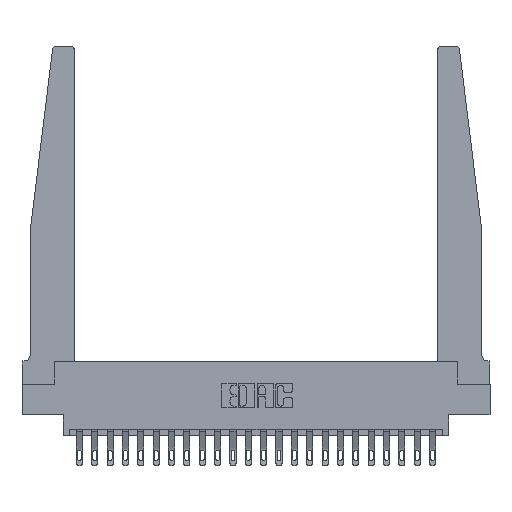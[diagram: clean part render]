
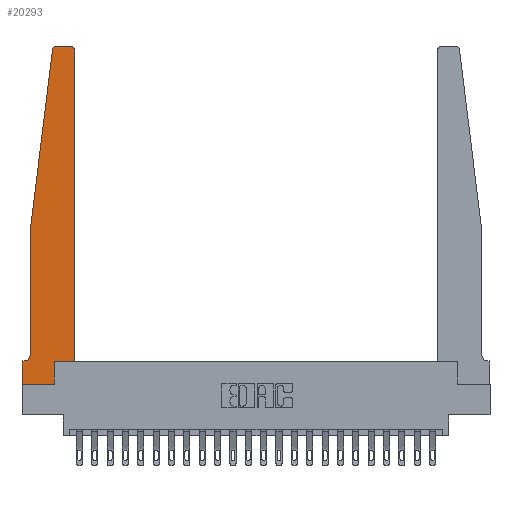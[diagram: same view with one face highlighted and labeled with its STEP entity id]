
A CAD part, top view. The second image highlights one B-rep face of the part: STEP entity #20293.
In plain terms, the highlighted planar face has unit normal (0, 0, 1).
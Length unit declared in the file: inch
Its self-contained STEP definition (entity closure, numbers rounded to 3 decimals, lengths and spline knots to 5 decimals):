
#299 = CIRCLE ( 'NONE', #3217, 0.03 ) ;
#361 = ORIENTED_EDGE ( 'NONE', *, *, #21332, .T. ) ;
#588 = VECTOR ( 'NONE', #3275, 39.37008 ) ;
#765 = LINE ( 'NONE', #5804, #19380 ) ;
#890 = EDGE_CURVE ( 'NONE', #10286, #17745, #2139, .T. ) ;
#1192 = VERTEX_POINT ( 'NONE', #19790 ) ;
#1317 = LINE ( 'NONE', #15060, #19360 ) ;
#1356 = AXIS2_PLACEMENT_3D ( 'NONE', #9595, #22176, #11411 ) ;
#1451 = DIRECTION ( 'NONE',  ( 0., 0., 1. ) ) ;
#1475 = CARTESIAN_POINT ( 'NONE',  ( 0.065, 1.25, 0.37 ) ) ;
#1739 = CARTESIAN_POINT ( 'NONE',  ( 0.425, 0.18, 0.37 ) ) ;
#1819 = ORIENTED_EDGE ( 'NONE', *, *, #6641, .T. ) ;
#1929 = CARTESIAN_POINT ( 'NONE',  ( 0.395, 2.75, 0.37 ) ) ;
#2139 = CIRCLE ( 'NONE', #16858, 0.05 ) ;
#3217 = AXIS2_PLACEMENT_3D ( 'NONE', #12265, #1451, #14056 ) ;
#3275 = DIRECTION ( 'NONE',  ( 0., -1., 0. ) ) ;
#3302 = CARTESIAN_POINT ( 'NONE',  ( 0.25, 2.75, 0.37 ) ) ;
#3959 = CARTESIAN_POINT ( 'NONE',  ( 0.065, 1.25, 0.37 ) ) ;
#4139 = CARTESIAN_POINT ( 'NONE',  ( 0.065, 0.2375, 0.37 ) ) ;
#4265 = DIRECTION ( 'NONE',  ( 0., 0., -1. ) ) ;
#4546 = EDGE_CURVE ( 'NONE', #10987, #20849, #12715, .T. ) ;
#4805 = ORIENTED_EDGE ( 'NONE', *, *, #10720, .T. ) ;
#4909 = VERTEX_POINT ( 'NONE', #11086 ) ;
#4997 = CARTESIAN_POINT ( 'NONE',  ( 0.27653, 2.75, 0.37 ) ) ;
#5639 = EDGE_LOOP ( 'NONE', ( #9806, #10664, #12303, #15102, #15524, #12689, #11533, #22842, #361, #4805, #1819, #17310 ) ) ;
#5682 = LINE ( 'NONE', #3302, #18344 ) ;
#5761 = LINE ( 'NONE', #9422, #9961 ) ;
#5804 = CARTESIAN_POINT ( 'NONE',  ( 0.2605, 0.18, 0.37 ) ) ;
#6040 = CARTESIAN_POINT ( 'NONE',  ( 0.2605, 0., 0.37 ) ) ;
#6432 = VECTOR ( 'NONE', #16168, 39.37008 ) ;
#6503 = CARTESIAN_POINT ( 'NONE',  ( 0., 0., 0.37 ) ) ;
#6641 = EDGE_CURVE ( 'NONE', #4909, #10987, #19247, .T. ) ;
#6982 = LINE ( 'NONE', #1739, #6432 ) ;
#7587 = DIRECTION ( 'NONE',  ( 0., 1., 0. ) ) ;
#7610 = EDGE_CURVE ( 'NONE', #13910, #10286, #20336, .T. ) ;
#7675 = DIRECTION ( 'NONE',  ( -1., 0., 0. ) ) ;
#7813 = DIRECTION ( 'NONE',  ( 0., 1., 0. ) ) ;
#7872 = DIRECTION ( 'NONE',  ( 1., 0., 0. ) ) ;
#8083 = LINE ( 'NONE', #10936, #17113 ) ;
#8285 = VERTEX_POINT ( 'NONE', #10668 ) ;
#8315 = CARTESIAN_POINT ( 'NONE',  ( 0., 0.1875, 0.37 ) ) ;
#8373 = AXIS2_PLACEMENT_3D ( 'NONE', #20166, #21979, #11200 ) ;
#9387 = PLANE ( 'NONE',  #8373 ) ;
#9422 = CARTESIAN_POINT ( 'NONE',  ( 0.065, 0.1875, 0.37 ) ) ;
#9595 = CARTESIAN_POINT ( 'NONE',  ( 0.395, 2.72, 0.37 ) ) ;
#9806 = ORIENTED_EDGE ( 'NONE', *, *, #16970, .T. ) ;
#9961 = VECTOR ( 'NONE', #7675, 39.37008 ) ;
#10286 = VERTEX_POINT ( 'NONE', #4139 ) ;
#10481 = EDGE_CURVE ( 'NONE', #23001, #1192, #15727, .T. ) ;
#10664 = ORIENTED_EDGE ( 'NONE', *, *, #19477, .T. ) ;
#10668 = CARTESIAN_POINT ( 'NONE',  ( 0.2605, 0.18, 0.37 ) ) ;
#10720 = EDGE_CURVE ( 'NONE', #8285, #4909, #6982, .T. ) ;
#10936 = CARTESIAN_POINT ( 'NONE',  ( 0.065, 1.25, 0.37 ) ) ;
#10953 = VECTOR ( 'NONE', #17280, 39.37008 ) ;
#10987 = VERTEX_POINT ( 'NONE', #22205 ) ;
#11037 = EDGE_CURVE ( 'NONE', #1192, #12130, #1317, .T. ) ;
#11086 = CARTESIAN_POINT ( 'NONE',  ( 0.425, 0.18, 0.37 ) ) ;
#11200 = DIRECTION ( 'NONE',  ( 1., 0., 0. ) ) ;
#11411 = DIRECTION ( 'NONE',  ( 1., 0., 0. ) ) ;
#11533 = ORIENTED_EDGE ( 'NONE', *, *, #10481, .T. ) ;
#11819 = DIRECTION ( 'NONE',  ( -1., 0., 0. ) ) ;
#11968 = VERTEX_POINT ( 'NONE', #16357 ) ;
#12130 = VERTEX_POINT ( 'NONE', #6040 ) ;
#12265 = CARTESIAN_POINT ( 'NONE',  ( 0.27653, 2.72, 0.37 ) ) ;
#12303 = ORIENTED_EDGE ( 'NONE', *, *, #22668, .T. ) ;
#12689 = ORIENTED_EDGE ( 'NONE', *, *, #15106, .T. ) ;
#12715 = CIRCLE ( 'NONE', #1356, 0.03 ) ;
#12812 = CARTESIAN_POINT ( 'NONE',  ( 0.015, 0.1875, 0.37 ) ) ;
#13910 = VERTEX_POINT ( 'NONE', #3959 ) ;
#14056 = DIRECTION ( 'NONE',  ( 1., 0., 0. ) ) ;
#14623 = DIRECTION ( 'NONE',  ( -0.122, -0.992, 0. ) ) ;
#15060 = CARTESIAN_POINT ( 'NONE',  ( 0., 0., 0.37 ) ) ;
#15102 = ORIENTED_EDGE ( 'NONE', *, *, #7610, .T. ) ;
#15106 = EDGE_CURVE ( 'NONE', #17745, #23001, #5761, .T. ) ;
#15524 = ORIENTED_EDGE ( 'NONE', *, *, #890, .T. ) ;
#15727 = LINE ( 'NONE', #6503, #10953 ) ;
#16168 = DIRECTION ( 'NONE',  ( 1., 0., 0. ) ) ;
#16357 = CARTESIAN_POINT ( 'NONE',  ( 0.24675, 2.72367, 0.37 ) ) ;
#16858 = AXIS2_PLACEMENT_3D ( 'NONE', #17617, #4265, #11819 ) ;
#16970 = EDGE_CURVE ( 'NONE', #20849, #18189, #5682, .T. ) ;
#17113 = VECTOR ( 'NONE', #14623, 39.37008 ) ;
#17280 = DIRECTION ( 'NONE',  ( 0., -1., 0. ) ) ;
#17310 = ORIENTED_EDGE ( 'NONE', *, *, #4546, .T. ) ;
#17476 = FACE_OUTER_BOUND ( 'NONE', #5639, .T. ) ;
#17617 = CARTESIAN_POINT ( 'NONE',  ( 0.015, 0.2375, 0.37 ) ) ;
#17742 = DIRECTION ( 'NONE',  ( -1., 0., 0. ) ) ;
#17745 = VERTEX_POINT ( 'NONE', #12812 ) ;
#18189 = VERTEX_POINT ( 'NONE', #4997 ) ;
#18344 = VECTOR ( 'NONE', #17742, 39.37008 ) ;
#18684 = VECTOR ( 'NONE', #7813, 39.37008 ) ;
#19247 = LINE ( 'NONE', #20419, #18684 ) ;
#19360 = VECTOR ( 'NONE', #7872, 39.37008 ) ;
#19380 = VECTOR ( 'NONE', #7587, 39.37008 ) ;
#19477 = EDGE_CURVE ( 'NONE', #18189, #11968, #299, .T. ) ;
#19790 = CARTESIAN_POINT ( 'NONE',  ( 0., 0., 0.37 ) ) ;
#20166 = CARTESIAN_POINT ( 'NONE',  ( 0., 0.1875, 0.37 ) ) ;
#20293 = ADVANCED_FACE ( 'NONE', ( #17476 ), #9387, .T. ) ;
#20336 = LINE ( 'NONE', #1475, #588 ) ;
#20419 = CARTESIAN_POINT ( 'NONE',  ( 0.425, 0.18, 0.37 ) ) ;
#20849 = VERTEX_POINT ( 'NONE', #1929 ) ;
#21332 = EDGE_CURVE ( 'NONE', #12130, #8285, #765, .T. ) ;
#21979 = DIRECTION ( 'NONE',  ( 0., 0., 1. ) ) ;
#22176 = DIRECTION ( 'NONE',  ( 0., 0., 1. ) ) ;
#22205 = CARTESIAN_POINT ( 'NONE',  ( 0.425, 2.72, 0.37 ) ) ;
#22668 = EDGE_CURVE ( 'NONE', #11968, #13910, #8083, .T. ) ;
#22842 = ORIENTED_EDGE ( 'NONE', *, *, #11037, .T. ) ;
#23001 = VERTEX_POINT ( 'NONE', #8315 ) ;
